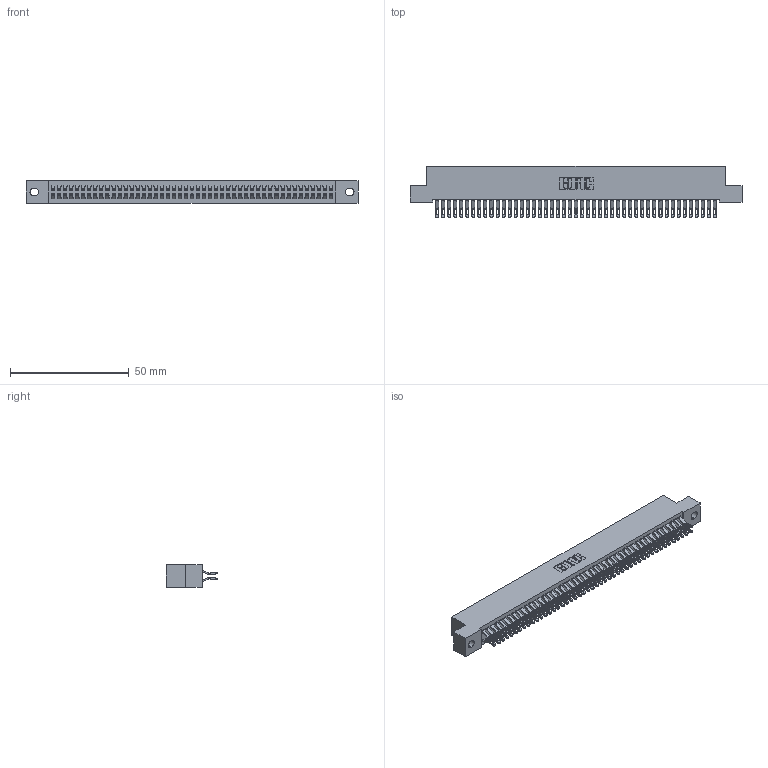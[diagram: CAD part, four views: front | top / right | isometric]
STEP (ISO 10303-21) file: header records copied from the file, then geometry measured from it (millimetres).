
FILE_DESCRIPTION (( 'STEP AP203' ), '1' );
FILE_NAME ('392-094-555-202.STEP', '2018-08-18T09:08:10', ( '' ), ( '' ), 'SwSTEP 2.0', 'SolidWorks 2016', '' );
FILE_SCHEMA (( 'CONFIG_CONTROL_DESIGN' ));
Length unit declared in the file: inch
Products named in the file (3): 342 Part_.128 Slot; 345-292-001_555 Tail; 392-094-555-202
Assembly tree (95 placements, depth 2):
  392-094-555-202
    342 Part_.128 Slot
    345-292-001_555 Tail  x94
Bounding box: 139.7 x 21.47 x 9.4 mm (x, y, z)
Volume: 12784.8 mm3; surface area: 21602.6 mm2
Topology: 95 solids, 95 shells, 5566 faces, 17513 edges, 11674 vertices
Faces by surface type: plane 3266, cylinder 2300
Entity records: 29919 total; most frequent: CARTESIAN_POINT 4988, ORIENTED_EDGE 4894, DIRECTION 4223, EDGE_CURVE 2447, LINE 2299, VECTOR 2299, VERTEX_POINT 1630, AXIS2_PLACEMENT_3D 962
